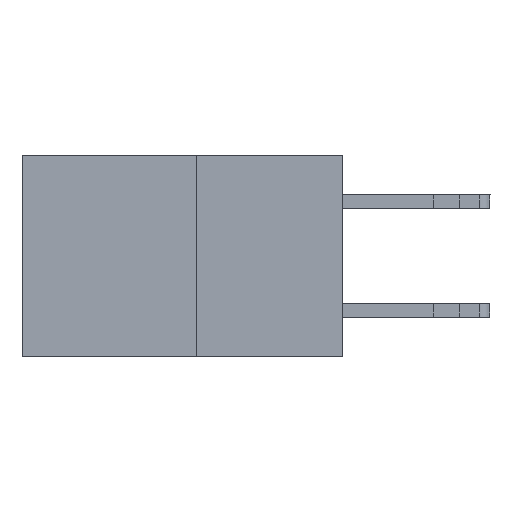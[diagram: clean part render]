
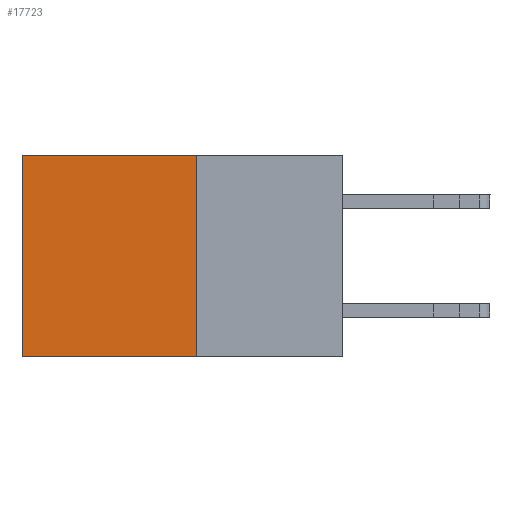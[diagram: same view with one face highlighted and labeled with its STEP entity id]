
A CAD part, left-side view. The second image highlights one B-rep face of the part: STEP entity #17723.
In plain terms, the highlighted planar face has unit normal (-1, 0, 0).
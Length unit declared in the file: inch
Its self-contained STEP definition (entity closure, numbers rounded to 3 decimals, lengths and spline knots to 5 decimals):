
#1412 = EDGE_CURVE ( 'NONE', #14759, #14453, #22533, .T. ) ;
#1588 = ORIENTED_EDGE ( 'NONE', *, *, #1412, .F. ) ;
#1613 = CARTESIAN_POINT ( 'NONE',  ( 0.277, 0.27, -0.37 ) ) ;
#2038 = CARTESIAN_POINT ( 'NONE',  ( 0.277, 0.27, 0. ) ) ;
#3952 = VECTOR ( 'NONE', #21843, 39.37008 ) ;
#4282 = EDGE_CURVE ( 'NONE', #9535, #14453, #8427, .T. ) ;
#5277 = PLANE ( 'NONE',  #18419 ) ;
#5398 = FACE_OUTER_BOUND ( 'NONE', #7594, .T. ) ;
#5477 = ORIENTED_EDGE ( 'NONE', *, *, #4282, .T. ) ;
#5547 = VECTOR ( 'NONE', #16482, 39.37008 ) ;
#6328 = DIRECTION ( 'NONE',  ( 0., 1., 0. ) ) ;
#6421 = DIRECTION ( 'NONE',  ( 0., 0., -1. ) ) ;
#7007 = ORIENTED_EDGE ( 'NONE', *, *, #7189, .F. ) ;
#7189 = EDGE_CURVE ( 'NONE', #18102, #14759, #8847, .T. ) ;
#7270 = DIRECTION ( 'NONE',  ( 1., 0., 0. ) ) ;
#7594 = EDGE_LOOP ( 'NONE', ( #5477, #1588, #7007, #10997 ) ) ;
#8191 = CARTESIAN_POINT ( 'NONE',  ( 0.277, 0.59, -0.37 ) ) ;
#8427 = LINE ( 'NONE', #8191, #17621 ) ;
#8847 = LINE ( 'NONE', #16180, #3952 ) ;
#9136 = CARTESIAN_POINT ( 'NONE',  ( 0.277, 0.59, 0. ) ) ;
#9535 = VERTEX_POINT ( 'NONE', #9136 ) ;
#10495 = VECTOR ( 'NONE', #6328, 39.37008 ) ;
#10997 = ORIENTED_EDGE ( 'NONE', *, *, #16765, .T. ) ;
#12493 = DIRECTION ( 'NONE',  ( 0., 0., -1. ) ) ;
#13545 = CARTESIAN_POINT ( 'NONE',  ( 0.277, 0.27, 0. ) ) ;
#13893 = CARTESIAN_POINT ( 'NONE',  ( 0.277, 0.27, -0.37 ) ) ;
#14453 = VERTEX_POINT ( 'NONE', #15526 ) ;
#14759 = VERTEX_POINT ( 'NONE', #1613 ) ;
#15526 = CARTESIAN_POINT ( 'NONE',  ( 0.277, 0.59, -0.37 ) ) ;
#16180 = CARTESIAN_POINT ( 'NONE',  ( 0.277, 0.27, -0.37 ) ) ;
#16482 = DIRECTION ( 'NONE',  ( 0., 1., 0. ) ) ;
#16765 = EDGE_CURVE ( 'NONE', #18102, #9535, #21574, .T. ) ;
#17621 = VECTOR ( 'NONE', #6421, 39.37008 ) ;
#17723 = ADVANCED_FACE ( 'NONE', ( #5398 ), #5277, .F. ) ;
#18038 = CARTESIAN_POINT ( 'NONE',  ( 0.277, 0.27, -0.37 ) ) ;
#18102 = VERTEX_POINT ( 'NONE', #13545 ) ;
#18419 = AXIS2_PLACEMENT_3D ( 'NONE', #18038, #7270, #12493 ) ;
#21574 = LINE ( 'NONE', #2038, #5547 ) ;
#21843 = DIRECTION ( 'NONE',  ( 0., 0., -1. ) ) ;
#22533 = LINE ( 'NONE', #13893, #10495 ) ;
